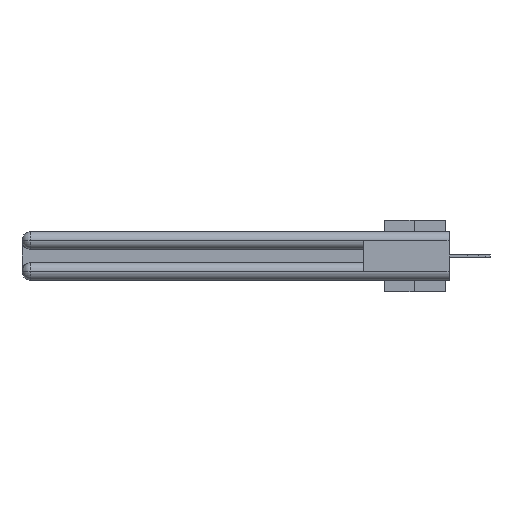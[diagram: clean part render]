
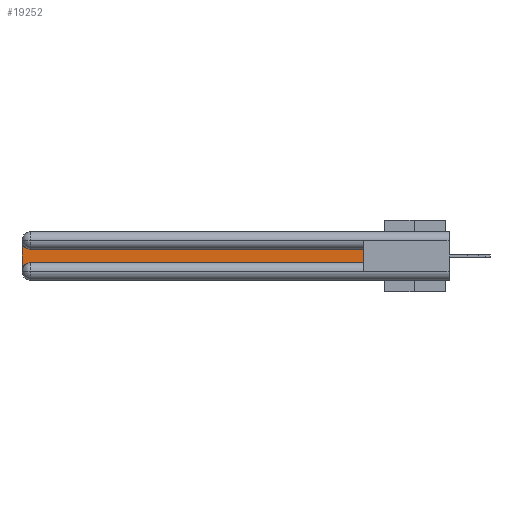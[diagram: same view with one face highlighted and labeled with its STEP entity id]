
A CAD part, left-side view. The second image highlights one B-rep face of the part: STEP entity #19252.
In plain terms, the highlighted planar face has unit normal (-1, 0, 0).
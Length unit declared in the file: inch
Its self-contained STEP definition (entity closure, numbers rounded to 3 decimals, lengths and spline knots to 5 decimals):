
#3631 = CARTESIAN_POINT ( 'NONE',  ( 0.075, 2.94, -0.2175 ) ) ;
#4039 = DIRECTION ( 'NONE',  ( 0., 0., -1. ) ) ;
#4383 = VECTOR ( 'NONE', #4039, 39.37008 ) ;
#5710 = EDGE_CURVE ( 'NONE', #19670, #9059, #18262, .T. ) ;
#5795 = CARTESIAN_POINT ( 'NONE',  ( 0.075, 0.6, -0.1225 ) ) ;
#6398 = EDGE_LOOP ( 'NONE', ( #28649, #16031, #12735, #25131, #6619, #9175 ) ) ;
#6619 = ORIENTED_EDGE ( 'NONE', *, *, #12026, .T. ) ;
#6674 = CARTESIAN_POINT ( 'NONE',  ( 0.075, 0.6, -0.2175 ) ) ;
#7820 = AXIS2_PLACEMENT_3D ( 'NONE', #16639, #28719, #11869 ) ;
#8480 = LINE ( 'NONE', #6674, #15810 ) ;
#8542 = AXIS2_PLACEMENT_3D ( 'NONE', #16794, #12170, #9295 ) ;
#9059 = VERTEX_POINT ( 'NONE', #19459 ) ;
#9175 = ORIENTED_EDGE ( 'NONE', *, *, #28444, .T. ) ;
#9295 = DIRECTION ( 'NONE',  ( 0., 0., -1. ) ) ;
#9797 = FACE_OUTER_BOUND ( 'NONE', #6398, .T. ) ;
#9939 = PLANE ( 'NONE',  #13109 ) ;
#10251 = LINE ( 'NONE', #24889, #12101 ) ;
#10570 = DIRECTION ( 'NONE',  ( 0., 0., 1. ) ) ;
#11214 = VERTEX_POINT ( 'NONE', #27984 ) ;
#11869 = DIRECTION ( 'NONE',  ( 0., 0., -1. ) ) ;
#12026 = EDGE_CURVE ( 'NONE', #23977, #31397, #8480, .T. ) ;
#12101 = VECTOR ( 'NONE', #10570, 39.37008 ) ;
#12170 = DIRECTION ( 'NONE',  ( 1., 0., 0. ) ) ;
#12735 = ORIENTED_EDGE ( 'NONE', *, *, #27801, .T. ) ;
#13109 = AXIS2_PLACEMENT_3D ( 'NONE', #24437, #17127, #26804 ) ;
#14403 = CARTESIAN_POINT ( 'NONE',  ( 0.075, 3., -0.2775 ) ) ;
#15552 = DIRECTION ( 'NONE',  ( 0., 1., 0. ) ) ;
#15810 = VECTOR ( 'NONE', #18222, 39.37008 ) ;
#16031 = ORIENTED_EDGE ( 'NONE', *, *, #20650, .T. ) ;
#16639 = CARTESIAN_POINT ( 'NONE',  ( 0.075, 2.94, -0.0625 ) ) ;
#16794 = CARTESIAN_POINT ( 'NONE',  ( 0.075, 2.94, -0.2775 ) ) ;
#17127 = DIRECTION ( 'NONE',  ( 1., 0., 0. ) ) ;
#17511 = CIRCLE ( 'NONE', #7820, 0.06 ) ;
#18222 = DIRECTION ( 'NONE',  ( 0., -1., 0. ) ) ;
#18262 = LINE ( 'NONE', #5795, #19943 ) ;
#19252 = ADVANCED_FACE ( 'NONE', ( #9797 ), #9939, .F. ) ;
#19459 = CARTESIAN_POINT ( 'NONE',  ( 0.075, 2.94, -0.1225 ) ) ;
#19670 = VERTEX_POINT ( 'NONE', #24683 ) ;
#19943 = VECTOR ( 'NONE', #15552, 39.37008 ) ;
#20650 = EDGE_CURVE ( 'NONE', #9059, #11214, #17511, .T. ) ;
#21781 = CIRCLE ( 'NONE', #8542, 0.06 ) ;
#23977 = VERTEX_POINT ( 'NONE', #3631 ) ;
#24437 = CARTESIAN_POINT ( 'NONE',  ( 0.075, 3., -0.1225 ) ) ;
#24683 = CARTESIAN_POINT ( 'NONE',  ( 0.075, 0.6, -0.1225 ) ) ;
#24889 = CARTESIAN_POINT ( 'NONE',  ( 0.075, 0.6, -0.2175 ) ) ;
#25131 = ORIENTED_EDGE ( 'NONE', *, *, #28798, .T. ) ;
#25723 = CARTESIAN_POINT ( 'NONE',  ( 0.075, 3., -0.2175 ) ) ;
#26804 = DIRECTION ( 'NONE',  ( 0., 0., -1. ) ) ;
#27249 = CARTESIAN_POINT ( 'NONE',  ( 0.075, 0.6, -0.2175 ) ) ;
#27801 = EDGE_CURVE ( 'NONE', #11214, #30420, #30994, .T. ) ;
#27984 = CARTESIAN_POINT ( 'NONE',  ( 0.075, 3., -0.0625 ) ) ;
#28444 = EDGE_CURVE ( 'NONE', #31397, #19670, #10251, .T. ) ;
#28649 = ORIENTED_EDGE ( 'NONE', *, *, #5710, .T. ) ;
#28719 = DIRECTION ( 'NONE',  ( 1., 0., 0. ) ) ;
#28798 = EDGE_CURVE ( 'NONE', #30420, #23977, #21781, .T. ) ;
#30420 = VERTEX_POINT ( 'NONE', #14403 ) ;
#30994 = LINE ( 'NONE', #25723, #4383 ) ;
#31397 = VERTEX_POINT ( 'NONE', #27249 ) ;
